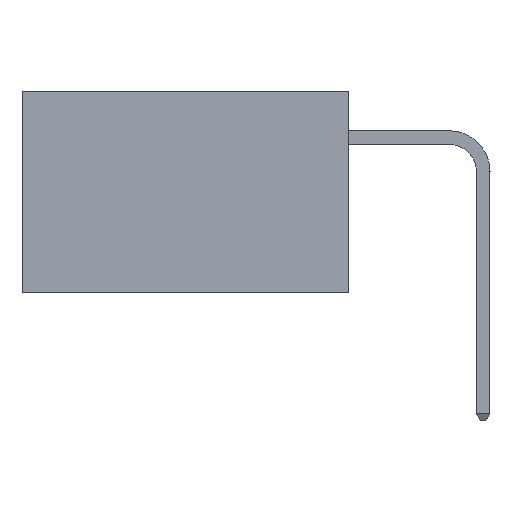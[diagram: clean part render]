
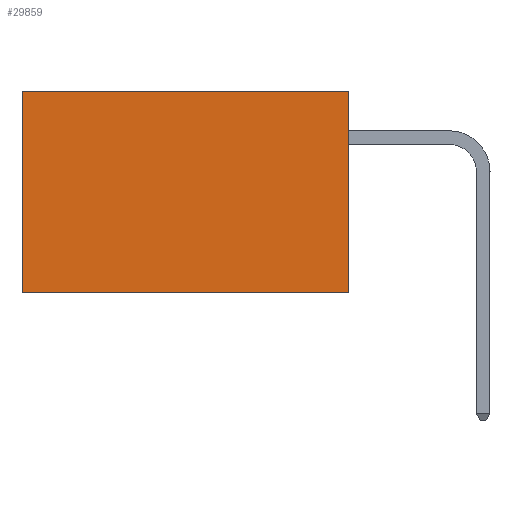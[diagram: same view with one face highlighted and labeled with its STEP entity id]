
A CAD part, left-side view. The second image highlights one B-rep face of the part: STEP entity #29859.
In plain terms, the highlighted planar face has unit normal (-1, 0, 0).
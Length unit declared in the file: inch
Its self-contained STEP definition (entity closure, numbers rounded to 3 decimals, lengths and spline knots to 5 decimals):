
#2974 = AXIS2_PLACEMENT_3D ( 'NONE', #28613, #31392, #14658 ) ;
#3690 = LINE ( 'NONE', #26960, #25240 ) ;
#3973 = VERTEX_POINT ( 'NONE', #27497 ) ;
#4331 = LINE ( 'NONE', #33550, #32343 ) ;
#4475 = EDGE_CURVE ( 'NONE', #21240, #27440, #3690, .T. ) ;
#5474 = CARTESIAN_POINT ( 'NONE',  ( 0.2875, 0., 0. ) ) ;
#5625 = ORIENTED_EDGE ( 'NONE', *, *, #34413, .T. ) ;
#7261 = DIRECTION ( 'NONE',  ( 0., 0., -1. ) ) ;
#7397 = DIRECTION ( 'NONE',  ( 0., 1., 0. ) ) ;
#7640 = CARTESIAN_POINT ( 'NONE',  ( 0.2875, 0.6, -0.37 ) ) ;
#7932 = CARTESIAN_POINT ( 'NONE',  ( 0.2875, 0., -0.37 ) ) ;
#8399 = DIRECTION ( 'NONE',  ( 0., 0., -1. ) ) ;
#8439 = ORIENTED_EDGE ( 'NONE', *, *, #8982, .T. ) ;
#8982 = EDGE_CURVE ( 'NONE', #3973, #17766, #4331, .T. ) ;
#11300 = CARTESIAN_POINT ( 'NONE',  ( 0.2875, 0., 0. ) ) ;
#11671 = ORIENTED_EDGE ( 'NONE', *, *, #21672, .F. ) ;
#14127 = DIRECTION ( 'NONE',  ( 0., 1., 0. ) ) ;
#14399 = ORIENTED_EDGE ( 'NONE', *, *, #4475, .F. ) ;
#14658 = DIRECTION ( 'NONE',  ( 0., 0., -1. ) ) ;
#17766 = VERTEX_POINT ( 'NONE', #7640 ) ;
#18009 = LINE ( 'NONE', #32450, #30205 ) ;
#19181 = FACE_OUTER_BOUND ( 'NONE', #33190, .T. ) ;
#21240 = VERTEX_POINT ( 'NONE', #5474 ) ;
#21672 = EDGE_CURVE ( 'NONE', #27440, #17766, #18009, .T. ) ;
#21738 = VECTOR ( 'NONE', #14127, 39.37008 ) ;
#25240 = VECTOR ( 'NONE', #7261, 39.37008 ) ;
#25841 = PLANE ( 'NONE',  #2974 ) ;
#26960 = CARTESIAN_POINT ( 'NONE',  ( 0.2875, 0., 0. ) ) ;
#27440 = VERTEX_POINT ( 'NONE', #7932 ) ;
#27497 = CARTESIAN_POINT ( 'NONE',  ( 0.2875, 0.6, 0. ) ) ;
#28613 = CARTESIAN_POINT ( 'NONE',  ( 0.2875, 0., 0. ) ) ;
#29859 = ADVANCED_FACE ( 'NONE', ( #19181 ), #25841, .F. ) ;
#29981 = LINE ( 'NONE', #11300, #21738 ) ;
#30205 = VECTOR ( 'NONE', #7397, 39.37008 ) ;
#31392 = DIRECTION ( 'NONE',  ( 1., 0., 0. ) ) ;
#32343 = VECTOR ( 'NONE', #8399, 39.37008 ) ;
#32450 = CARTESIAN_POINT ( 'NONE',  ( 0.2875, 0., -0.37 ) ) ;
#33190 = EDGE_LOOP ( 'NONE', ( #8439, #11671, #14399, #5625 ) ) ;
#33550 = CARTESIAN_POINT ( 'NONE',  ( 0.2875, 0.6, 0. ) ) ;
#34413 = EDGE_CURVE ( 'NONE', #21240, #3973, #29981, .T. ) ;
